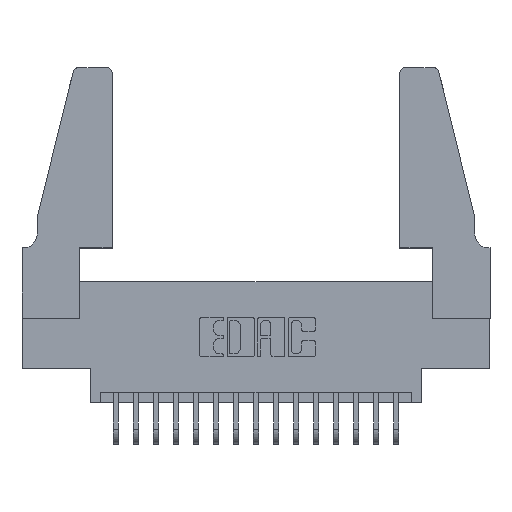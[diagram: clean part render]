
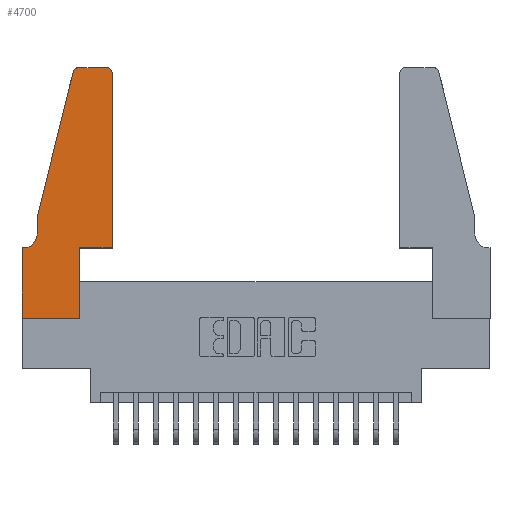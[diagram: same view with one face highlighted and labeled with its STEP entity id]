
A CAD part, top view. The second image highlights one B-rep face of the part: STEP entity #4700.
In plain terms, the highlighted planar face has unit normal (0, 0, 1).
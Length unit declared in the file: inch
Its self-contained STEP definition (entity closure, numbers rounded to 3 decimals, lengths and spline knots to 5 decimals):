
#307 = EDGE_CURVE ( 'NONE', #2246, #680, #4780, .T. ) ;
#443 = VERTEX_POINT ( 'NONE', #8402 ) ;
#680 = VERTEX_POINT ( 'NONE', #7659 ) ;
#750 = DIRECTION ( 'NONE',  ( 0., -1., 0. ) ) ;
#776 = ORIENTED_EDGE ( 'NONE', *, *, #7254, .T. ) ;
#1356 = ORIENTED_EDGE ( 'NONE', *, *, #307, .T. ) ;
#1377 = VECTOR ( 'NONE', #1715, 39.37008 ) ;
#1568 = ORIENTED_EDGE ( 'NONE', *, *, #4926, .T. ) ;
#1592 = DIRECTION ( 'NONE',  ( 0., 0., 1. ) ) ;
#1715 = DIRECTION ( 'NONE',  ( -1., 0., 0. ) ) ;
#1757 = CIRCLE ( 'NONE', #16161, 0.03 ) ;
#1771 = VECTOR ( 'NONE', #750, 39.37008 ) ;
#1774 = EDGE_LOOP ( 'NONE', ( #1568, #9485, #8834, #3734, #4930, #776, #19319, #10540, #12084, #11344, #14570, #1356 ) ) ;
#1838 = VECTOR ( 'NONE', #18967, 39.37008 ) ;
#2246 = VERTEX_POINT ( 'NONE', #3999 ) ;
#2261 = VECTOR ( 'NONE', #9686, 39.37008 ) ;
#2296 = VERTEX_POINT ( 'NONE', #7616 ) ;
#2332 = VERTEX_POINT ( 'NONE', #5337 ) ;
#2399 = AXIS2_PLACEMENT_3D ( 'NONE', #3598, #16888, #7953 ) ;
#2482 = LINE ( 'NONE', #9741, #14677 ) ;
#2832 = EDGE_CURVE ( 'NONE', #3158, #2296, #1757, .T. ) ;
#3158 = VERTEX_POINT ( 'NONE', #13021 ) ;
#3598 = CARTESIAN_POINT ( 'NONE',  ( 0.4205, 1.22, 0.37 ) ) ;
#3734 = ORIENTED_EDGE ( 'NONE', *, *, #6287, .T. ) ;
#3999 = CARTESIAN_POINT ( 'NONE',  ( 0.4505, 1.22, 0.37 ) ) ;
#4369 = CARTESIAN_POINT ( 'NONE',  ( 0.4505, 0.35, 0.37 ) ) ;
#4493 = CARTESIAN_POINT ( 'NONE',  ( 0., 0., 0.37 ) ) ;
#4623 = VERTEX_POINT ( 'NONE', #6078 ) ;
#4700 = ADVANCED_FACE ( 'NONE', ( #16933 ), #5892, .T. ) ;
#4780 = CIRCLE ( 'NONE', #2399, 0.03 ) ;
#4874 = CARTESIAN_POINT ( 'NONE',  ( 0.284, 1.22, 0.37 ) ) ;
#4926 = EDGE_CURVE ( 'NONE', #680, #3158, #13176, .T. ) ;
#4930 = ORIENTED_EDGE ( 'NONE', *, *, #17018, .T. ) ;
#5313 = CARTESIAN_POINT ( 'NONE',  ( 0., 0., 0.37 ) ) ;
#5337 = CARTESIAN_POINT ( 'NONE',  ( 0.0755, 0.42, 0.37 ) ) ;
#5892 = PLANE ( 'NONE',  #15912 ) ;
#6078 = CARTESIAN_POINT ( 'NONE',  ( 0.0055, 0.35, 0.37 ) ) ;
#6193 = CARTESIAN_POINT ( 'NONE',  ( 0., 0.35, 0.37 ) ) ;
#6287 = EDGE_CURVE ( 'NONE', #15431, #2332, #7306, .T. ) ;
#6326 = LINE ( 'NONE', #6805, #1838 ) ;
#6334 = CARTESIAN_POINT ( 'NONE',  ( 0.2865, 0., 0.37 ) ) ;
#6405 = VECTOR ( 'NONE', #19288, 39.37008 ) ;
#6573 = CARTESIAN_POINT ( 'NONE',  ( 0.2605, 1.25, 0.37 ) ) ;
#6633 = DIRECTION ( 'NONE',  ( 0., -1., 0. ) ) ;
#6745 = CARTESIAN_POINT ( 'NONE',  ( 0., 0., 0.37 ) ) ;
#6805 = CARTESIAN_POINT ( 'NONE',  ( 0.0755, 0.5, 0.37 ) ) ;
#6864 = DIRECTION ( 'NONE',  ( 0., 1., 0. ) ) ;
#6896 = CARTESIAN_POINT ( 'NONE',  ( 0.0755, 0.5, 0.37 ) ) ;
#7078 = EDGE_CURVE ( 'NONE', #2296, #15431, #6326, .T. ) ;
#7221 = VERTEX_POINT ( 'NONE', #4369 ) ;
#7254 = EDGE_CURVE ( 'NONE', #4623, #10236, #14232, .T. ) ;
#7306 = LINE ( 'NONE', #6896, #10320 ) ;
#7603 = CARTESIAN_POINT ( 'NONE',  ( 0.2865, 0.35, 0.37 ) ) ;
#7616 = CARTESIAN_POINT ( 'NONE',  ( 0.25487, 1.22718, 0.37 ) ) ;
#7659 = CARTESIAN_POINT ( 'NONE',  ( 0.4205, 1.25, 0.37 ) ) ;
#7953 = DIRECTION ( 'NONE',  ( 1., 0., 0. ) ) ;
#8168 = AXIS2_PLACEMENT_3D ( 'NONE', #13170, #19008, #17773 ) ;
#8366 = LINE ( 'NONE', #14155, #2261 ) ;
#8402 = CARTESIAN_POINT ( 'NONE',  ( 0.2865, 0.35, 0.37 ) ) ;
#8834 = ORIENTED_EDGE ( 'NONE', *, *, #7078, .T. ) ;
#9392 = CARTESIAN_POINT ( 'NONE',  ( 0.0755, 0.5, 0.37 ) ) ;
#9485 = ORIENTED_EDGE ( 'NONE', *, *, #2832, .T. ) ;
#9686 = DIRECTION ( 'NONE',  ( 1., 0., 0. ) ) ;
#9741 = CARTESIAN_POINT ( 'NONE',  ( 0.4505, 0.35, 0.37 ) ) ;
#10236 = VERTEX_POINT ( 'NONE', #6193 ) ;
#10320 = VECTOR ( 'NONE', #6633, 39.37008 ) ;
#10540 = ORIENTED_EDGE ( 'NONE', *, *, #12694, .T. ) ;
#10697 = CARTESIAN_POINT ( 'NONE',  ( 0.0755, 0.35, 0.37 ) ) ;
#11344 = ORIENTED_EDGE ( 'NONE', *, *, #12169, .T. ) ;
#11373 = LINE ( 'NONE', #5313, #1771 ) ;
#11390 = VECTOR ( 'NONE', #19166, 39.37008 ) ;
#11986 = CARTESIAN_POINT ( 'NONE',  ( 0., 0.35, 0.37 ) ) ;
#12047 = DIRECTION ( 'NONE',  ( 1., 0., 0. ) ) ;
#12069 = VECTOR ( 'NONE', #17898, 39.37008 ) ;
#12084 = ORIENTED_EDGE ( 'NONE', *, *, #15234, .T. ) ;
#12141 = EDGE_CURVE ( 'NONE', #7221, #2246, #2482, .T. ) ;
#12169 = EDGE_CURVE ( 'NONE', #443, #7221, #8366, .T. ) ;
#12694 = EDGE_CURVE ( 'NONE', #13777, #14938, #17717, .T. ) ;
#13021 = CARTESIAN_POINT ( 'NONE',  ( 0.284, 1.25, 0.37 ) ) ;
#13170 = CARTESIAN_POINT ( 'NONE',  ( 0.0055, 0.42, 0.37 ) ) ;
#13176 = LINE ( 'NONE', #6573, #6405 ) ;
#13777 = VERTEX_POINT ( 'NONE', #6745 ) ;
#14155 = CARTESIAN_POINT ( 'NONE',  ( 0.4505, 0.35, 0.37 ) ) ;
#14232 = LINE ( 'NONE', #10697, #1377 ) ;
#14570 = ORIENTED_EDGE ( 'NONE', *, *, #12141, .T. ) ;
#14677 = VECTOR ( 'NONE', #6864, 39.37008 ) ;
#14938 = VERTEX_POINT ( 'NONE', #6334 ) ;
#15234 = EDGE_CURVE ( 'NONE', #14938, #443, #15349, .T. ) ;
#15332 = DIRECTION ( 'NONE',  ( 0., 0., 1. ) ) ;
#15349 = LINE ( 'NONE', #7603, #11390 ) ;
#15431 = VERTEX_POINT ( 'NONE', #9392 ) ;
#15515 = EDGE_CURVE ( 'NONE', #10236, #13777, #11373, .T. ) ;
#15912 = AXIS2_PLACEMENT_3D ( 'NONE', #11986, #1592, #12047 ) ;
#16161 = AXIS2_PLACEMENT_3D ( 'NONE', #4874, #15332, #18346 ) ;
#16245 = CIRCLE ( 'NONE', #8168, 0.07 ) ;
#16888 = DIRECTION ( 'NONE',  ( 0., 0., 1. ) ) ;
#16933 = FACE_OUTER_BOUND ( 'NONE', #1774, .T. ) ;
#17018 = EDGE_CURVE ( 'NONE', #2332, #4623, #16245, .T. ) ;
#17717 = LINE ( 'NONE', #4493, #12069 ) ;
#17773 = DIRECTION ( 'NONE',  ( -1., 0., 0. ) ) ;
#17898 = DIRECTION ( 'NONE',  ( 1., 0., 0. ) ) ;
#18346 = DIRECTION ( 'NONE',  ( 1., 0., 0. ) ) ;
#18967 = DIRECTION ( 'NONE',  ( -0.239, -0.971, 0. ) ) ;
#19008 = DIRECTION ( 'NONE',  ( 0., 0., -1. ) ) ;
#19166 = DIRECTION ( 'NONE',  ( 0., 1., 0. ) ) ;
#19288 = DIRECTION ( 'NONE',  ( -1., 0., 0. ) ) ;
#19319 = ORIENTED_EDGE ( 'NONE', *, *, #15515, .T. ) ;
